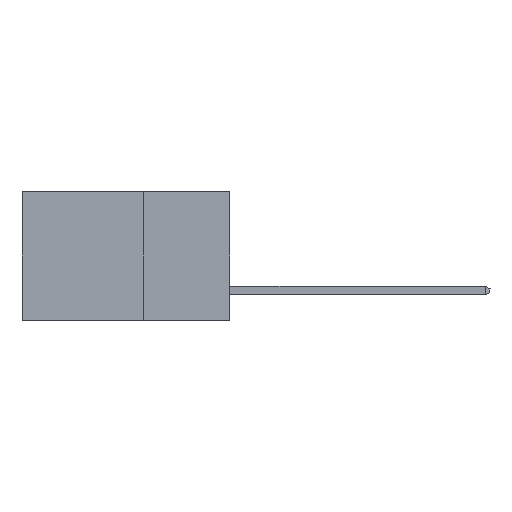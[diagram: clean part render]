
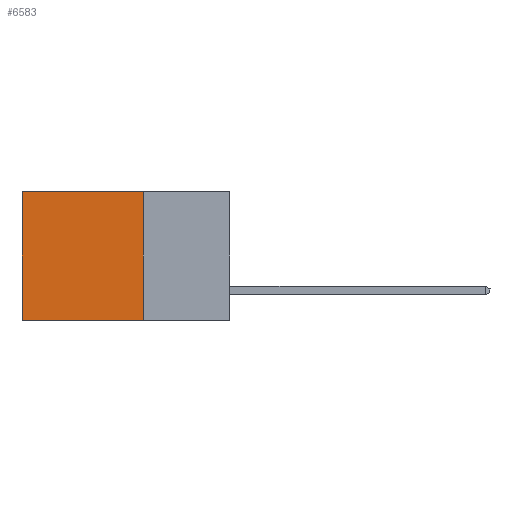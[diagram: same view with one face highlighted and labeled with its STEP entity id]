
A CAD part, left-side view. The second image highlights one B-rep face of the part: STEP entity #6583.
In plain terms, the highlighted planar face has unit normal (-1, 0, 0).
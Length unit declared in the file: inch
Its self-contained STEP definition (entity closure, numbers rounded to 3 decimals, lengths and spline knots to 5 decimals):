
#821 = DIRECTION ( 'NONE',  ( 0., 1., 0. ) ) ;
#824 = CARTESIAN_POINT ( 'NONE',  ( 0.298, 0.6, -0.37 ) ) ;
#851 = PLANE ( 'NONE',  #7913 ) ;
#1198 = CARTESIAN_POINT ( 'NONE',  ( 0.298, 0.25, 0. ) ) ;
#1306 = EDGE_LOOP ( 'NONE', ( #7197, #3704, #8556, #2329 ) ) ;
#1743 = DIRECTION ( 'NONE',  ( 0., 0., -1. ) ) ;
#1921 = CARTESIAN_POINT ( 'NONE',  ( 0.298, 0.25, 0. ) ) ;
#2156 = EDGE_CURVE ( 'NONE', #6894, #12489, #4589, .T. ) ;
#2329 = ORIENTED_EDGE ( 'NONE', *, *, #2156, .T. ) ;
#2336 = DIRECTION ( 'NONE',  ( 0., 0., -1. ) ) ;
#2494 = VERTEX_POINT ( 'NONE', #824 ) ;
#3186 = CARTESIAN_POINT ( 'NONE',  ( 0.298, 0.25, 0. ) ) ;
#3704 = ORIENTED_EDGE ( 'NONE', *, *, #8741, .F. ) ;
#4219 = FACE_OUTER_BOUND ( 'NONE', #1306, .T. ) ;
#4322 = DIRECTION ( 'NONE',  ( 0., 1., 0. ) ) ;
#4512 = VECTOR ( 'NONE', #2336, 39.37008 ) ;
#4589 = LINE ( 'NONE', #1198, #7607 ) ;
#5905 = EDGE_CURVE ( 'NONE', #12489, #2494, #6650, .T. ) ;
#5995 = CARTESIAN_POINT ( 'NONE',  ( 0.298, 0.25, -0.37 ) ) ;
#6096 = LINE ( 'NONE', #5995, #11162 ) ;
#6583 = ADVANCED_FACE ( 'NONE', ( #4219 ), #851, .F. ) ;
#6650 = LINE ( 'NONE', #10923, #10748 ) ;
#6894 = VERTEX_POINT ( 'NONE', #12914 ) ;
#7091 = DIRECTION ( 'NONE',  ( 0., 0., -1. ) ) ;
#7197 = ORIENTED_EDGE ( 'NONE', *, *, #5905, .T. ) ;
#7500 = EDGE_CURVE ( 'NONE', #6894, #10678, #11989, .T. ) ;
#7607 = VECTOR ( 'NONE', #4322, 39.37008 ) ;
#7707 = CARTESIAN_POINT ( 'NONE',  ( 0.298, 0.25, -0.37 ) ) ;
#7913 = AXIS2_PLACEMENT_3D ( 'NONE', #1921, #12132, #7091 ) ;
#8556 = ORIENTED_EDGE ( 'NONE', *, *, #7500, .F. ) ;
#8741 = EDGE_CURVE ( 'NONE', #10678, #2494, #6096, .T. ) ;
#9052 = CARTESIAN_POINT ( 'NONE',  ( 0.298, 0.6, 0. ) ) ;
#10678 = VERTEX_POINT ( 'NONE', #7707 ) ;
#10748 = VECTOR ( 'NONE', #1743, 39.37008 ) ;
#10923 = CARTESIAN_POINT ( 'NONE',  ( 0.298, 0.6, 0. ) ) ;
#11162 = VECTOR ( 'NONE', #821, 39.37008 ) ;
#11989 = LINE ( 'NONE', #3186, #4512 ) ;
#12132 = DIRECTION ( 'NONE',  ( 1., 0., 0. ) ) ;
#12489 = VERTEX_POINT ( 'NONE', #9052 ) ;
#12914 = CARTESIAN_POINT ( 'NONE',  ( 0.298, 0.25, 0. ) ) ;
